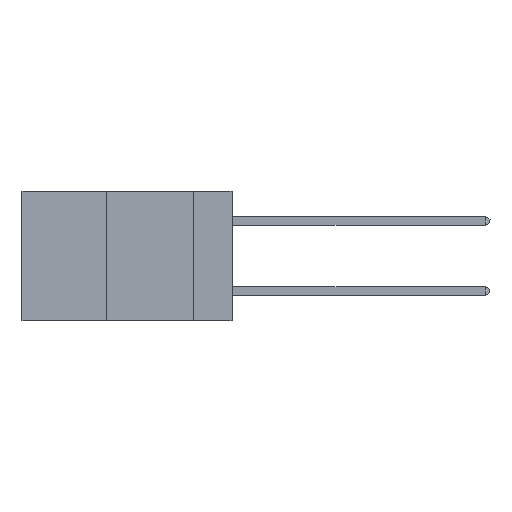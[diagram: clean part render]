
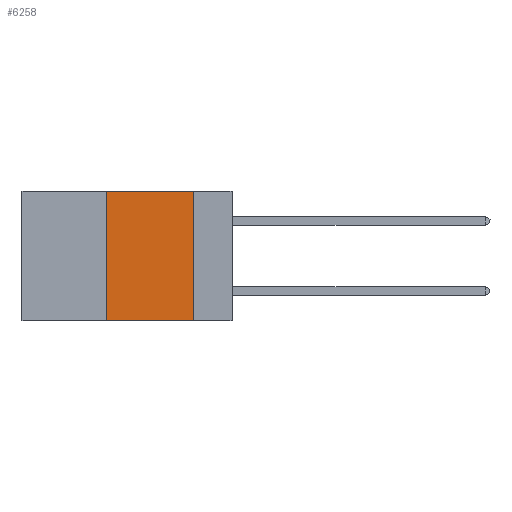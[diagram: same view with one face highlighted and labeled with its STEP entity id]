
A CAD part, left-side view. The second image highlights one B-rep face of the part: STEP entity #6258.
In plain terms, the highlighted planar face has unit normal (-1, 0, 0).
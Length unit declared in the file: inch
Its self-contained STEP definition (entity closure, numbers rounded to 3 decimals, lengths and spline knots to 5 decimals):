
#1050 = CARTESIAN_POINT ( 'NONE',  ( 0., 0.11, 0. ) ) ;
#3040 = ORIENTED_EDGE ( 'NONE', *, *, #23215, .F. ) ;
#5262 = CARTESIAN_POINT ( 'NONE',  ( 0., 0.11, 0. ) ) ;
#5645 = CARTESIAN_POINT ( 'NONE',  ( 0., 0.6, 0. ) ) ;
#6094 = EDGE_CURVE ( 'NONE', #9089, #23229, #37510, .T. ) ;
#6258 = ADVANCED_FACE ( 'NONE', ( #35106 ), #25604, .F. ) ;
#6497 = EDGE_CURVE ( 'NONE', #9089, #24738, #20041, .T. ) ;
#7035 = AXIS2_PLACEMENT_3D ( 'NONE', #22228, #28864, #22370 ) ;
#7147 = CARTESIAN_POINT ( 'NONE',  ( 0., 0.36, -0.37 ) ) ;
#7821 = DIRECTION ( 'NONE',  ( 0., 0., 1. ) ) ;
#9089 = VERTEX_POINT ( 'NONE', #7147 ) ;
#10025 = DIRECTION ( 'NONE',  ( 0., 0., -1. ) ) ;
#11816 = VECTOR ( 'NONE', #38220, 39.37008 ) ;
#11827 = DIRECTION ( 'NONE',  ( 0., -1., 0. ) ) ;
#12462 = ORIENTED_EDGE ( 'NONE', *, *, #6094, .F. ) ;
#13287 = EDGE_CURVE ( 'NONE', #23229, #15931, #15113, .T. ) ;
#14183 = VECTOR ( 'NONE', #11827, 39.37008 ) ;
#15113 = LINE ( 'NONE', #5645, #14183 ) ;
#15154 = LINE ( 'NONE', #1050, #34567 ) ;
#15931 = VERTEX_POINT ( 'NONE', #5262 ) ;
#16569 = CARTESIAN_POINT ( 'NONE',  ( 0., 0.36, 0. ) ) ;
#17423 = ORIENTED_EDGE ( 'NONE', *, *, #6497, .T. ) ;
#19016 = EDGE_LOOP ( 'NONE', ( #3040, #28407, #12462, #17423 ) ) ;
#20041 = LINE ( 'NONE', #34829, #11816 ) ;
#20075 = VECTOR ( 'NONE', #7821, 39.37008 ) ;
#22228 = CARTESIAN_POINT ( 'NONE',  ( 0., 0.6, 0. ) ) ;
#22370 = DIRECTION ( 'NONE',  ( 0., 0., -1. ) ) ;
#23215 = EDGE_CURVE ( 'NONE', #15931, #24738, #15154, .T. ) ;
#23229 = VERTEX_POINT ( 'NONE', #16569 ) ;
#24738 = VERTEX_POINT ( 'NONE', #34526 ) ;
#25604 = PLANE ( 'NONE',  #7035 ) ;
#28407 = ORIENTED_EDGE ( 'NONE', *, *, #13287, .F. ) ;
#28864 = DIRECTION ( 'NONE',  ( 1., 0., 0. ) ) ;
#34526 = CARTESIAN_POINT ( 'NONE',  ( 0., 0.11, -0.37 ) ) ;
#34567 = VECTOR ( 'NONE', #10025, 39.37008 ) ;
#34829 = CARTESIAN_POINT ( 'NONE',  ( 0., 0.6, -0.37 ) ) ;
#35106 = FACE_OUTER_BOUND ( 'NONE', #19016, .T. ) ;
#37510 = LINE ( 'NONE', #39876, #20075 ) ;
#38220 = DIRECTION ( 'NONE',  ( 0., -1., 0. ) ) ;
#39876 = CARTESIAN_POINT ( 'NONE',  ( 0., 0.36, 0. ) ) ;
